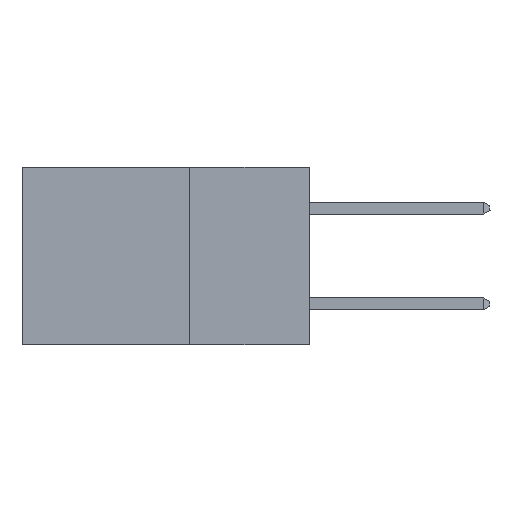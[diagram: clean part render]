
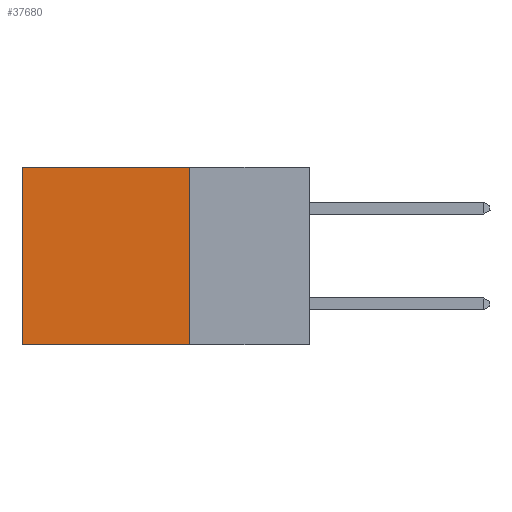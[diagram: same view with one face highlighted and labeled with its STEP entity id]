
A CAD part, left-side view. The second image highlights one B-rep face of the part: STEP entity #37680.
In plain terms, the highlighted planar face has unit normal (-1, 0, 0).
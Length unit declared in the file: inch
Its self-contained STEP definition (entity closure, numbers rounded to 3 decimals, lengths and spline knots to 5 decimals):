
#1374 = FACE_OUTER_BOUND ( 'NONE', #20418, .T. ) ;
#2345 = ORIENTED_EDGE ( 'NONE', *, *, #11093, .T. ) ;
#2517 = VECTOR ( 'NONE', #15047, 39.37008 ) ;
#5889 = CARTESIAN_POINT ( 'NONE',  ( 0.2875, 0.25, 0. ) ) ;
#7523 = VERTEX_POINT ( 'NONE', #5889 ) ;
#8788 = CARTESIAN_POINT ( 'NONE',  ( 0.2875, 0.6, 0. ) ) ;
#10144 = CARTESIAN_POINT ( 'NONE',  ( 0.2875, 0.6, 0. ) ) ;
#10256 = CARTESIAN_POINT ( 'NONE',  ( 0.2875, 0.25, -0.37 ) ) ;
#11093 = EDGE_CURVE ( 'NONE', #26847, #38191, #24658, .T. ) ;
#11406 = CARTESIAN_POINT ( 'NONE',  ( 0.2875, 0.25, 0. ) ) ;
#14237 = AXIS2_PLACEMENT_3D ( 'NONE', #11406, #39564, #18638 ) ;
#14832 = EDGE_CURVE ( 'NONE', #27975, #38191, #19258, .T. ) ;
#14844 = DIRECTION ( 'NONE',  ( 0., 1., 0. ) ) ;
#14993 = VECTOR ( 'NONE', #14844, 39.37008 ) ;
#15047 = DIRECTION ( 'NONE',  ( 0., 0., -1. ) ) ;
#15128 = VECTOR ( 'NONE', #21733, 39.37008 ) ;
#15479 = ORIENTED_EDGE ( 'NONE', *, *, #23473, .T. ) ;
#17966 = CARTESIAN_POINT ( 'NONE',  ( 0.2875, 0.25, 0. ) ) ;
#18638 = DIRECTION ( 'NONE',  ( 0., 0., -1. ) ) ;
#19258 = LINE ( 'NONE', #10256, #31864 ) ;
#20418 = EDGE_LOOP ( 'NONE', ( #2345, #38544, #25878, #15479 ) ) ;
#21112 = LINE ( 'NONE', #30871, #2517 ) ;
#21733 = DIRECTION ( 'NONE',  ( 0., 0., -1. ) ) ;
#23473 = EDGE_CURVE ( 'NONE', #7523, #26847, #24847, .T. ) ;
#24658 = LINE ( 'NONE', #8788, #15128 ) ;
#24847 = LINE ( 'NONE', #17966, #14993 ) ;
#25878 = ORIENTED_EDGE ( 'NONE', *, *, #29254, .F. ) ;
#26847 = VERTEX_POINT ( 'NONE', #10144 ) ;
#27748 = CARTESIAN_POINT ( 'NONE',  ( 0.2875, 0.6, -0.37 ) ) ;
#27975 = VERTEX_POINT ( 'NONE', #36743 ) ;
#29254 = EDGE_CURVE ( 'NONE', #7523, #27975, #21112, .T. ) ;
#30871 = CARTESIAN_POINT ( 'NONE',  ( 0.2875, 0.25, 0. ) ) ;
#31864 = VECTOR ( 'NONE', #34700, 39.37008 ) ;
#34476 = PLANE ( 'NONE',  #14237 ) ;
#34700 = DIRECTION ( 'NONE',  ( 0., 1., 0. ) ) ;
#36743 = CARTESIAN_POINT ( 'NONE',  ( 0.2875, 0.25, -0.37 ) ) ;
#37680 = ADVANCED_FACE ( 'NONE', ( #1374 ), #34476, .F. ) ;
#38191 = VERTEX_POINT ( 'NONE', #27748 ) ;
#38544 = ORIENTED_EDGE ( 'NONE', *, *, #14832, .F. ) ;
#39564 = DIRECTION ( 'NONE',  ( 1., 0., 0. ) ) ;
